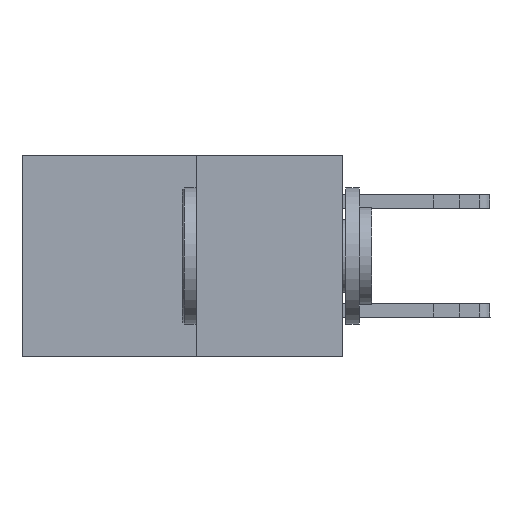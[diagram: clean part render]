
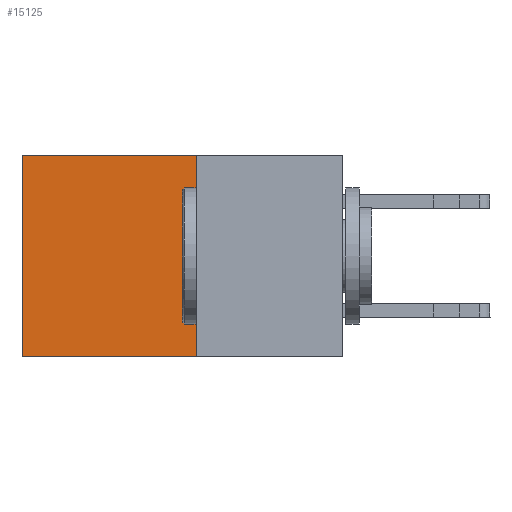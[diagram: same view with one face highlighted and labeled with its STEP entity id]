
A CAD part, left-side view. The second image highlights one B-rep face of the part: STEP entity #15125.
In plain terms, the highlighted planar face has unit normal (-1, 0, 0).
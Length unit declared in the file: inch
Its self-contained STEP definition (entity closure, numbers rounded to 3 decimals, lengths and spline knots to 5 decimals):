
#178 = VERTEX_POINT ( 'NONE', #16803 ) ;
#1739 = LINE ( 'NONE', #7220, #10434 ) ;
#2315 = CARTESIAN_POINT ( 'NONE',  ( 0.277, 0.27, 0. ) ) ;
#4529 = EDGE_CURVE ( 'NONE', #16979, #178, #17572, .T. ) ;
#6276 = ORIENTED_EDGE ( 'NONE', *, *, #16819, .T. ) ;
#6612 = FACE_OUTER_BOUND ( 'NONE', #17199, .T. ) ;
#6677 = LINE ( 'NONE', #18372, #15273 ) ;
#7220 = CARTESIAN_POINT ( 'NONE',  ( 0.277, 0.59, -0.37 ) ) ;
#7432 = DIRECTION ( 'NONE',  ( 0., 1., 0. ) ) ;
#7869 = PLANE ( 'NONE',  #20411 ) ;
#8428 = VECTOR ( 'NONE', #12763, 39.37008 ) ;
#8924 = DIRECTION ( 'NONE',  ( 0., 0., -1. ) ) ;
#10434 = VECTOR ( 'NONE', #8924, 39.37008 ) ;
#11191 = VERTEX_POINT ( 'NONE', #19099 ) ;
#11303 = DIRECTION ( 'NONE',  ( 0., 0., -1. ) ) ;
#12525 = CARTESIAN_POINT ( 'NONE',  ( 0.277, 0.27, -0.37 ) ) ;
#12581 = VERTEX_POINT ( 'NONE', #14078 ) ;
#12763 = DIRECTION ( 'NONE',  ( 0., 0., -1. ) ) ;
#12825 = VECTOR ( 'NONE', #7432, 39.37008 ) ;
#13381 = LINE ( 'NONE', #21095, #12825 ) ;
#13751 = EDGE_CURVE ( 'NONE', #178, #12581, #6677, .T. ) ;
#14078 = CARTESIAN_POINT ( 'NONE',  ( 0.277, 0.59, -0.37 ) ) ;
#15125 = ADVANCED_FACE ( 'NONE', ( #6612 ), #7869, .F. ) ;
#15273 = VECTOR ( 'NONE', #20070, 39.37008 ) ;
#16803 = CARTESIAN_POINT ( 'NONE',  ( 0.277, 0.27, -0.37 ) ) ;
#16819 = EDGE_CURVE ( 'NONE', #11191, #12581, #1739, .T. ) ;
#16928 = EDGE_CURVE ( 'NONE', #16979, #11191, #13381, .T. ) ;
#16979 = VERTEX_POINT ( 'NONE', #2315 ) ;
#17199 = EDGE_LOOP ( 'NONE', ( #6276, #19399, #17407, #19889 ) ) ;
#17407 = ORIENTED_EDGE ( 'NONE', *, *, #4529, .F. ) ;
#17572 = LINE ( 'NONE', #12525, #8428 ) ;
#18372 = CARTESIAN_POINT ( 'NONE',  ( 0.277, 0.27, -0.37 ) ) ;
#19099 = CARTESIAN_POINT ( 'NONE',  ( 0.277, 0.59, 0. ) ) ;
#19399 = ORIENTED_EDGE ( 'NONE', *, *, #13751, .F. ) ;
#19863 = CARTESIAN_POINT ( 'NONE',  ( 0.277, 0.27, -0.37 ) ) ;
#19889 = ORIENTED_EDGE ( 'NONE', *, *, #16928, .T. ) ;
#20070 = DIRECTION ( 'NONE',  ( 0., 1., 0. ) ) ;
#20411 = AXIS2_PLACEMENT_3D ( 'NONE', #19863, #21598, #11303 ) ;
#21095 = CARTESIAN_POINT ( 'NONE',  ( 0.277, 0.27, 0. ) ) ;
#21598 = DIRECTION ( 'NONE',  ( 1., 0., 0. ) ) ;
